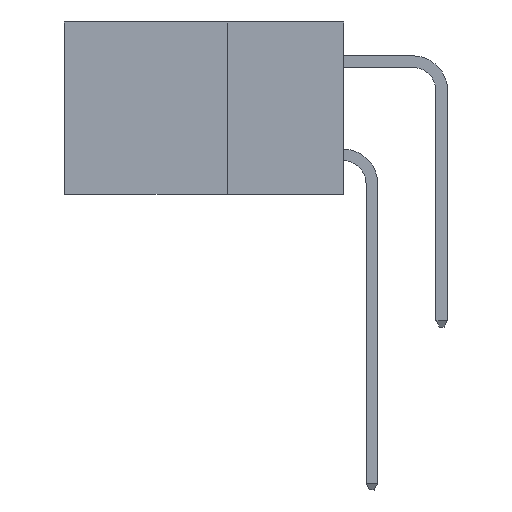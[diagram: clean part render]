
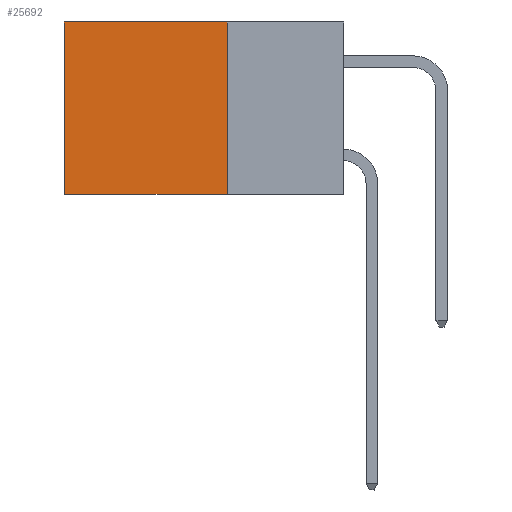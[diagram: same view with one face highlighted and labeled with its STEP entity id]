
A CAD part, left-side view. The second image highlights one B-rep face of the part: STEP entity #25692.
In plain terms, the highlighted planar face has unit normal (-1, 0, 0).
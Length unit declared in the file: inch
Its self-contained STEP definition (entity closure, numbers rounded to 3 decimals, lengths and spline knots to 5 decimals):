
#137 = VERTEX_POINT ( 'NONE', #19305 ) ;
#610 = LINE ( 'NONE', #25837, #15697 ) ;
#1109 = EDGE_CURVE ( 'NONE', #18871, #26722, #610, .T. ) ;
#1974 = DIRECTION ( 'NONE',  ( 0., 0., -1. ) ) ;
#2128 = CARTESIAN_POINT ( 'NONE',  ( 0.298, 0.25, 0. ) ) ;
#3706 = VECTOR ( 'NONE', #8929, 39.37008 ) ;
#4513 = LINE ( 'NONE', #6168, #3706 ) ;
#5760 = CARTESIAN_POINT ( 'NONE',  ( 0.298, 0.6, 0. ) ) ;
#6125 = AXIS2_PLACEMENT_3D ( 'NONE', #2128, #29947, #24967 ) ;
#6168 = CARTESIAN_POINT ( 'NONE',  ( 0.298, 0.25, 0. ) ) ;
#8002 = DIRECTION ( 'NONE',  ( 0., 0., -1. ) ) ;
#8929 = DIRECTION ( 'NONE',  ( 0., 1., 0. ) ) ;
#9232 = ORIENTED_EDGE ( 'NONE', *, *, #1109, .F. ) ;
#9769 = PLANE ( 'NONE',  #6125 ) ;
#10098 = DIRECTION ( 'NONE',  ( 0., 1., 0. ) ) ;
#10396 = CARTESIAN_POINT ( 'NONE',  ( 0.298, 0.6, -0.37 ) ) ;
#12039 = EDGE_CURVE ( 'NONE', #29682, #26722, #13482, .T. ) ;
#12065 = CARTESIAN_POINT ( 'NONE',  ( 0.298, 0.6, 0. ) ) ;
#12649 = VECTOR ( 'NONE', #8002, 39.37008 ) ;
#12727 = ORIENTED_EDGE ( 'NONE', *, *, #12039, .T. ) ;
#13349 = FACE_OUTER_BOUND ( 'NONE', #27979, .T. ) ;
#13482 = LINE ( 'NONE', #12065, #27073 ) ;
#13649 = EDGE_CURVE ( 'NONE', #137, #18871, #28992, .T. ) ;
#15697 = VECTOR ( 'NONE', #10098, 39.37008 ) ;
#18505 = ORIENTED_EDGE ( 'NONE', *, *, #21432, .T. ) ;
#18871 = VERTEX_POINT ( 'NONE', #24091 ) ;
#19305 = CARTESIAN_POINT ( 'NONE',  ( 0.298, 0.25, 0. ) ) ;
#21432 = EDGE_CURVE ( 'NONE', #137, #29682, #4513, .T. ) ;
#23645 = CARTESIAN_POINT ( 'NONE',  ( 0.298, 0.25, 0. ) ) ;
#24091 = CARTESIAN_POINT ( 'NONE',  ( 0.298, 0.25, -0.37 ) ) ;
#24967 = DIRECTION ( 'NONE',  ( 0., 0., -1. ) ) ;
#25692 = ADVANCED_FACE ( 'NONE', ( #13349 ), #9769, .F. ) ;
#25837 = CARTESIAN_POINT ( 'NONE',  ( 0.298, 0.25, -0.37 ) ) ;
#26722 = VERTEX_POINT ( 'NONE', #10396 ) ;
#27073 = VECTOR ( 'NONE', #1974, 39.37008 ) ;
#27979 = EDGE_LOOP ( 'NONE', ( #12727, #9232, #31151, #18505 ) ) ;
#28992 = LINE ( 'NONE', #23645, #12649 ) ;
#29682 = VERTEX_POINT ( 'NONE', #5760 ) ;
#29947 = DIRECTION ( 'NONE',  ( 1., 0., 0. ) ) ;
#31151 = ORIENTED_EDGE ( 'NONE', *, *, #13649, .F. ) ;
